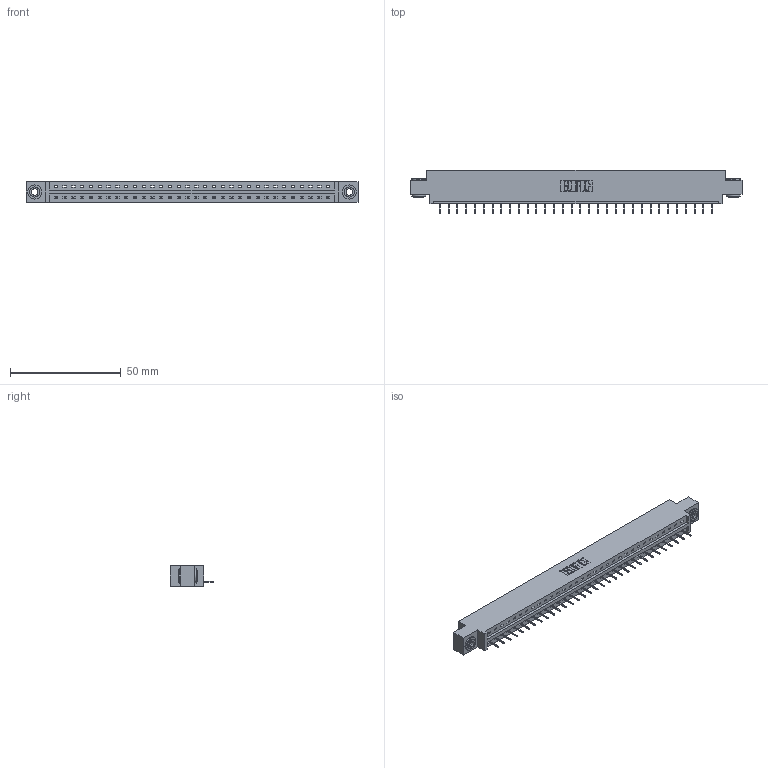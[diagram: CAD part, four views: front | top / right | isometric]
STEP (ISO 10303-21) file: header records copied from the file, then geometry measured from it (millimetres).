
FILE_DESCRIPTION (( 'STEP AP203' ), '1' );
FILE_NAME ('337-032-524-603.STEP', '2018-08-07T05:29:39', ( '' ), ( '' ), 'SwSTEP 2.0', 'SolidWorks 2016', '' );
FILE_SCHEMA (( 'CONFIG_CONTROL_DESIGN' ));
Length unit declared in the file: inch
Products named in the file (4): 337-032-524-603; 337 Part_0.170 Offset - 0.156 Dia-TH; 345-292-001_345-293-124; 345-250-002_345-250-002-102
Assembly tree (35 placements, depth 2):
  337-032-524-603
    337 Part_0.170 Offset - 0.156 Dia-TH
    345-292-001_345-293-124  x32
    345-250-002_345-250-002-102  x2
Bounding box: 149.81 x 19.69 x 9.4 mm (x, y, z)
Volume: 15220.5 mm3; surface area: 15557.2 mm2
Topology: 35 solids, 35 shells, 2268 faces, 6543 edges, 4230 vertices
Faces by surface type: plane 1748, cylinder 512, cone 8
Entity records: 25936 total; most frequent: CARTESIAN_POINT 4493, ORIENTED_EDGE 4454, DIRECTION 3837, EDGE_CURVE 2227, VECTOR 2079, LINE 2079, VERTEX_POINT 1478, AXIS2_PLACEMENT_3D 879
